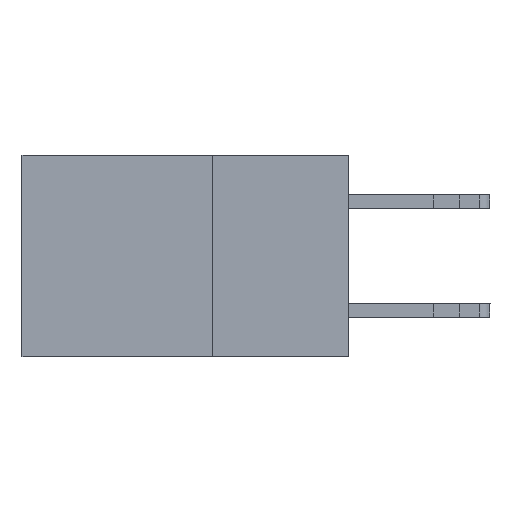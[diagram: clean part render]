
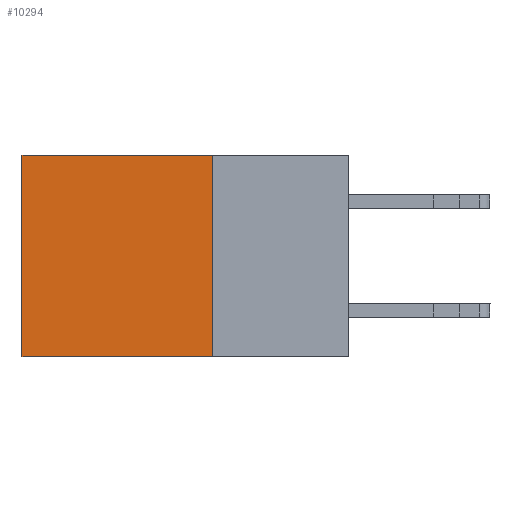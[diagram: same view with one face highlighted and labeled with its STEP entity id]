
A CAD part, left-side view. The second image highlights one B-rep face of the part: STEP entity #10294.
In plain terms, the highlighted planar face has unit normal (-1, 0, 0).
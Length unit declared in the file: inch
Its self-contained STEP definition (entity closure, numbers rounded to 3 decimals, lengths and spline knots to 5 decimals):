
#612 = CARTESIAN_POINT ( 'NONE',  ( 0.2615, 0.25, 0. ) ) ;
#641 = ORIENTED_EDGE ( 'NONE', *, *, #6161, .T. ) ;
#677 = DIRECTION ( 'NONE',  ( 0., 1., 0. ) ) ;
#875 = LINE ( 'NONE', #6414, #6021 ) ;
#943 = ORIENTED_EDGE ( 'NONE', *, *, #11186, .T. ) ;
#2512 = DIRECTION ( 'NONE',  ( 0., 0., -1. ) ) ;
#3214 = DIRECTION ( 'NONE',  ( 0., 0., -1. ) ) ;
#3355 = VERTEX_POINT ( 'NONE', #7621 ) ;
#3770 = DIRECTION ( 'NONE',  ( 0., 0., -1. ) ) ;
#3774 = ORIENTED_EDGE ( 'NONE', *, *, #7962, .F. ) ;
#4054 = VECTOR ( 'NONE', #8898, 39.37008 ) ;
#4183 = LINE ( 'NONE', #8007, #4054 ) ;
#4288 = CARTESIAN_POINT ( 'NONE',  ( 0.2615, 0.6, 0. ) ) ;
#5005 = DIRECTION ( 'NONE',  ( 1., 0., 0. ) ) ;
#5948 = CARTESIAN_POINT ( 'NONE',  ( 0.2615, 0.25, -0.37 ) ) ;
#6016 = VECTOR ( 'NONE', #677, 39.37008 ) ;
#6021 = VECTOR ( 'NONE', #3770, 39.37008 ) ;
#6038 = CARTESIAN_POINT ( 'NONE',  ( 0.2615, 0.25, -0.37 ) ) ;
#6161 = EDGE_CURVE ( 'NONE', #10882, #8101, #875, .T. ) ;
#6162 = FACE_OUTER_BOUND ( 'NONE', #6241, .T. ) ;
#6241 = EDGE_LOOP ( 'NONE', ( #641, #8912, #3774, #943 ) ) ;
#6414 = CARTESIAN_POINT ( 'NONE',  ( 0.2615, 0.6, -0.37 ) ) ;
#7621 = CARTESIAN_POINT ( 'NONE',  ( 0.2615, 0.25, -0.37 ) ) ;
#7633 = VERTEX_POINT ( 'NONE', #8190 ) ;
#7897 = LINE ( 'NONE', #612, #6016 ) ;
#7962 = EDGE_CURVE ( 'NONE', #7633, #3355, #10276, .T. ) ;
#8007 = CARTESIAN_POINT ( 'NONE',  ( 0.2615, 0.25, -0.37 ) ) ;
#8101 = VERTEX_POINT ( 'NONE', #8758 ) ;
#8190 = CARTESIAN_POINT ( 'NONE',  ( 0.2615, 0.25, 0. ) ) ;
#8523 = VECTOR ( 'NONE', #2512, 39.37008 ) ;
#8758 = CARTESIAN_POINT ( 'NONE',  ( 0.2615, 0.6, -0.37 ) ) ;
#8898 = DIRECTION ( 'NONE',  ( 0., 1., 0. ) ) ;
#8912 = ORIENTED_EDGE ( 'NONE', *, *, #10138, .F. ) ;
#9266 = PLANE ( 'NONE',  #10801 ) ;
#10138 = EDGE_CURVE ( 'NONE', #3355, #8101, #4183, .T. ) ;
#10276 = LINE ( 'NONE', #6038, #8523 ) ;
#10294 = ADVANCED_FACE ( 'NONE', ( #6162 ), #9266, .F. ) ;
#10801 = AXIS2_PLACEMENT_3D ( 'NONE', #5948, #5005, #3214 ) ;
#10882 = VERTEX_POINT ( 'NONE', #4288 ) ;
#11186 = EDGE_CURVE ( 'NONE', #7633, #10882, #7897, .T. ) ;
